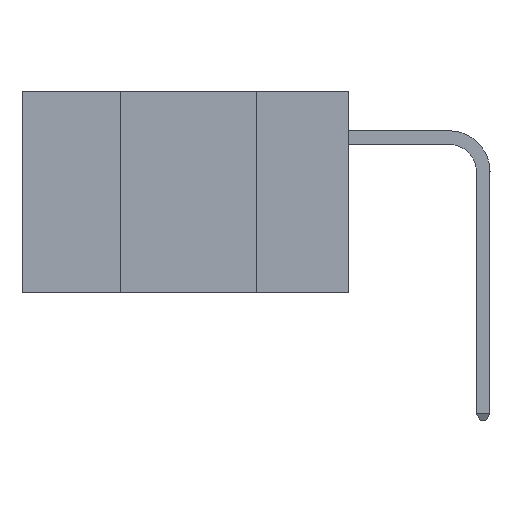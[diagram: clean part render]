
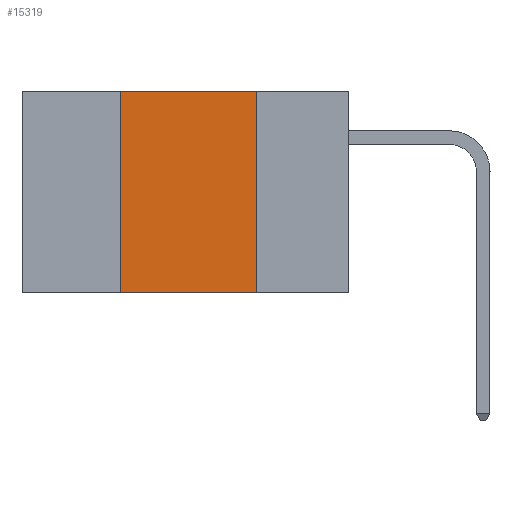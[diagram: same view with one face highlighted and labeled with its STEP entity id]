
A CAD part, left-side view. The second image highlights one B-rep face of the part: STEP entity #15319.
In plain terms, the highlighted planar face has unit normal (-1, 0, 0).
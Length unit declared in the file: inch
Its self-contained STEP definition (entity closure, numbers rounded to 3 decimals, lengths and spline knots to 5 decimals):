
#203 = VERTEX_POINT ( 'NONE', #8577 ) ;
#1147 = EDGE_CURVE ( 'NONE', #17779, #19872, #32697, .T. ) ;
#1985 = EDGE_LOOP ( 'NONE', ( #14436, #30772, #33485, #36167 ) ) ;
#3674 = CARTESIAN_POINT ( 'NONE',  ( 0., 0.17, 0. ) ) ;
#5105 = EDGE_CURVE ( 'NONE', #203, #17779, #5334, .T. ) ;
#5334 = LINE ( 'NONE', #29125, #34389 ) ;
#5718 = CARTESIAN_POINT ( 'NONE',  ( 0., 0.6, -0.37 ) ) ;
#6698 = LINE ( 'NONE', #5718, #21276 ) ;
#6945 = PLANE ( 'NONE',  #16496 ) ;
#7287 = DIRECTION ( 'NONE',  ( 0., 0., 1. ) ) ;
#8012 = LINE ( 'NONE', #27624, #31167 ) ;
#8577 = CARTESIAN_POINT ( 'NONE',  ( 0., 0.42, 0. ) ) ;
#9327 = FACE_OUTER_BOUND ( 'NONE', #1985, .T. ) ;
#12716 = EDGE_CURVE ( 'NONE', #26233, #19872, #6698, .T. ) ;
#12805 = DIRECTION ( 'NONE',  ( 0., 0., -1. ) ) ;
#13118 = CARTESIAN_POINT ( 'NONE',  ( 0., 0.17, -0.37 ) ) ;
#13900 = CARTESIAN_POINT ( 'NONE',  ( 0., 0.17, 0. ) ) ;
#14436 = ORIENTED_EDGE ( 'NONE', *, *, #1147, .F. ) ;
#14764 = DIRECTION ( 'NONE',  ( 0., -1., 0. ) ) ;
#15319 = ADVANCED_FACE ( 'NONE', ( #9327 ), #6945, .F. ) ;
#16496 = AXIS2_PLACEMENT_3D ( 'NONE', #32948, #30178, #12805 ) ;
#17779 = VERTEX_POINT ( 'NONE', #3674 ) ;
#19872 = VERTEX_POINT ( 'NONE', #13118 ) ;
#21276 = VECTOR ( 'NONE', #31752, 39.37008 ) ;
#22697 = DIRECTION ( 'NONE',  ( 0., 0., -1. ) ) ;
#24133 = VECTOR ( 'NONE', #22697, 39.37008 ) ;
#26233 = VERTEX_POINT ( 'NONE', #31501 ) ;
#27624 = CARTESIAN_POINT ( 'NONE',  ( 0., 0.42, 0. ) ) ;
#29125 = CARTESIAN_POINT ( 'NONE',  ( 0., 0.6, 0. ) ) ;
#30178 = DIRECTION ( 'NONE',  ( 1., 0., 0. ) ) ;
#30772 = ORIENTED_EDGE ( 'NONE', *, *, #5105, .F. ) ;
#31167 = VECTOR ( 'NONE', #7287, 39.37008 ) ;
#31501 = CARTESIAN_POINT ( 'NONE',  ( 0., 0.42, -0.37 ) ) ;
#31752 = DIRECTION ( 'NONE',  ( 0., -1., 0. ) ) ;
#32697 = LINE ( 'NONE', #13900, #24133 ) ;
#32948 = CARTESIAN_POINT ( 'NONE',  ( 0., 0.6, 0. ) ) ;
#33485 = ORIENTED_EDGE ( 'NONE', *, *, #35763, .F. ) ;
#34389 = VECTOR ( 'NONE', #14764, 39.37008 ) ;
#35763 = EDGE_CURVE ( 'NONE', #26233, #203, #8012, .T. ) ;
#36167 = ORIENTED_EDGE ( 'NONE', *, *, #12716, .T. ) ;
